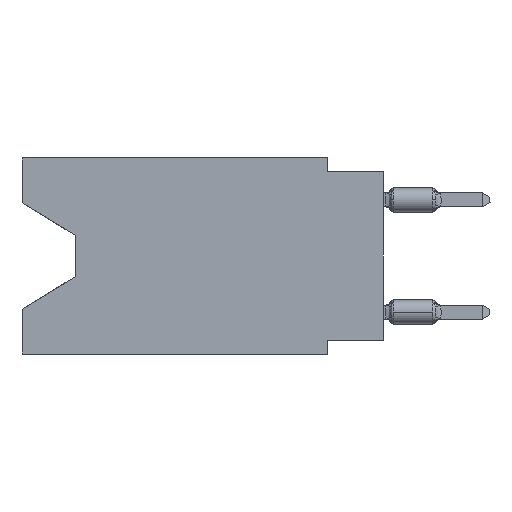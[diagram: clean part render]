
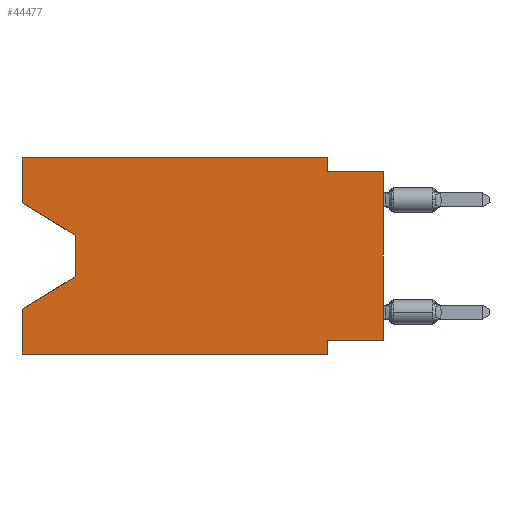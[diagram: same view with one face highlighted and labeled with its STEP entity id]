
A CAD part, left-side view. The second image highlights one B-rep face of the part: STEP entity #44477.
In plain terms, the highlighted planar face has unit normal (-1, 0, 0).
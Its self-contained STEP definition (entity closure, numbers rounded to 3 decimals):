
#53 = EDGE_CURVE ( 'NONE', #8936, #19838, #831, .T. ) ;
#192 = DIRECTION ( 'NONE',  ( 0., 0., 1. ) ) ;
#831 = LINE ( 'NONE', #1366, #6568 ) ;
#1353 = CARTESIAN_POINT ( 'NONE',  ( 0., 16.383, -2.038 ) ) ;
#1366 = CARTESIAN_POINT ( 'NONE',  ( 0., 16.383, -8.89 ) ) ;
#1413 = DIRECTION ( 'NONE',  ( 0., -1., 0. ) ) ;
#1794 = LINE ( 'NONE', #10398, #28857 ) ;
#2228 = VERTEX_POINT ( 'NONE', #4451 ) ;
#2782 = VERTEX_POINT ( 'NONE', #1353 ) ;
#2998 = DIRECTION ( 'NONE',  ( 0., 0., 1. ) ) ;
#3834 = FACE_OUTER_BOUND ( 'NONE', #28465, .T. ) ;
#4344 = VECTOR ( 'NONE', #18576, 1000. ) ;
#4451 = CARTESIAN_POINT ( 'NONE',  ( 0., 16.383, 0. ) ) ;
#4560 = LINE ( 'NONE', #53153, #26335 ) ;
#5319 = VECTOR ( 'NONE', #192, 1000. ) ;
#5365 = ORIENTED_EDGE ( 'NONE', *, *, #13552, .F. ) ;
#6349 = DIRECTION ( 'NONE',  ( 0., 0., -1. ) ) ;
#6568 = VECTOR ( 'NONE', #33372, 1000. ) ;
#6982 = VERTEX_POINT ( 'NONE', #52504 ) ;
#7954 = ORIENTED_EDGE ( 'NONE', *, *, #28000, .F. ) ;
#8135 = DIRECTION ( 'NONE',  ( 1., 0., 0. ) ) ;
#8501 = DIRECTION ( 'NONE',  ( 0., -1., 0. ) ) ;
#8926 = CARTESIAN_POINT ( 'NONE',  ( 0., 16.383, 0. ) ) ;
#8936 = VERTEX_POINT ( 'NONE', #34368 ) ;
#8953 = ORIENTED_EDGE ( 'NONE', *, *, #37714, .T. ) ;
#9332 = LINE ( 'NONE', #12830, #5319 ) ;
#10398 = CARTESIAN_POINT ( 'NONE',  ( 0., 2.54, -8.89 ) ) ;
#10589 = VECTOR ( 'NONE', #8501, 1000. ) ;
#11578 = CARTESIAN_POINT ( 'NONE',  ( 0., 13.97, -3.505 ) ) ;
#12590 = VERTEX_POINT ( 'NONE', #17169 ) ;
#12830 = CARTESIAN_POINT ( 'NONE',  ( 0., 16.383, 0. ) ) ;
#13552 = EDGE_CURVE ( 'NONE', #2782, #2228, #9332, .T. ) ;
#13594 = DIRECTION ( 'NONE',  ( 0., 0., -1. ) ) ;
#14296 = VERTEX_POINT ( 'NONE', #23752 ) ;
#14804 = ORIENTED_EDGE ( 'NONE', *, *, #40997, .F. ) ;
#15452 = ORIENTED_EDGE ( 'NONE', *, *, #26032, .T. ) ;
#15479 = CARTESIAN_POINT ( 'NONE',  ( 0., 13.97, -3.505 ) ) ;
#16416 = DIRECTION ( 'NONE',  ( 0., 0.855, -0.519 ) ) ;
#17169 = CARTESIAN_POINT ( 'NONE',  ( 0., 16.383, -6.852 ) ) ;
#17277 = PLANE ( 'NONE',  #29744 ) ;
#17378 = LINE ( 'NONE', #25703, #10589 ) ;
#17562 = LINE ( 'NONE', #26161, #45477 ) ;
#18576 = DIRECTION ( 'NONE',  ( 0., -0.855, -0.519 ) ) ;
#18681 = EDGE_CURVE ( 'NONE', #14296, #6982, #38583, .T. ) ;
#18889 = CARTESIAN_POINT ( 'NONE',  ( 0., 16.383, 0. ) ) ;
#19838 = VERTEX_POINT ( 'NONE', #30572 ) ;
#20214 = VERTEX_POINT ( 'NONE', #22178 ) ;
#20826 = EDGE_CURVE ( 'NONE', #35823, #30790, #28523, .T. ) ;
#21378 = ORIENTED_EDGE ( 'NONE', *, *, #30723, .F. ) ;
#22178 = CARTESIAN_POINT ( 'NONE',  ( 0., 0., -0.635 ) ) ;
#23124 = CARTESIAN_POINT ( 'NONE',  ( 0., 0., -8.255 ) ) ;
#23237 = ORIENTED_EDGE ( 'NONE', *, *, #18681, .F. ) ;
#23752 = CARTESIAN_POINT ( 'NONE',  ( 0., 2.54, 0. ) ) ;
#23971 = LINE ( 'NONE', #18889, #41963 ) ;
#25141 = EDGE_CURVE ( 'NONE', #2228, #14296, #17562, .T. ) ;
#25703 = CARTESIAN_POINT ( 'NONE',  ( 0., 0., -0.635 ) ) ;
#26032 = EDGE_CURVE ( 'NONE', #2782, #35823, #51874, .T. ) ;
#26161 = CARTESIAN_POINT ( 'NONE',  ( 0., 16.383, 0. ) ) ;
#26335 = VECTOR ( 'NONE', #16416, 1000. ) ;
#26837 = ORIENTED_EDGE ( 'NONE', *, *, #53, .T. ) ;
#26952 = VECTOR ( 'NONE', #41823, 1000. ) ;
#27309 = ORIENTED_EDGE ( 'NONE', *, *, #20826, .T. ) ;
#28000 = EDGE_CURVE ( 'NONE', #46604, #19838, #1794, .T. ) ;
#28158 = VECTOR ( 'NONE', #44898, 1000. ) ;
#28465 = EDGE_LOOP ( 'NONE', ( #15452, #27309, #51441, #14804, #26837, #7954, #21378, #8953, #45550, #23237, #42887, #5365 ) ) ;
#28523 = LINE ( 'NONE', #11578, #28158 ) ;
#28845 = DIRECTION ( 'NONE',  ( 0., 0., -1. ) ) ;
#28857 = VECTOR ( 'NONE', #6349, 1000. ) ;
#29477 = LINE ( 'NONE', #45852, #26952 ) ;
#29549 = VECTOR ( 'NONE', #34249, 1000. ) ;
#29744 = AXIS2_PLACEMENT_3D ( 'NONE', #8926, #8135, #28845 ) ;
#29955 = CARTESIAN_POINT ( 'NONE',  ( 0., 13.97, -5.385 ) ) ;
#30145 = EDGE_CURVE ( 'NONE', #6982, #20214, #17378, .T. ) ;
#30572 = CARTESIAN_POINT ( 'NONE',  ( 0., 2.54, -8.89 ) ) ;
#30664 = CARTESIAN_POINT ( 'NONE',  ( 0., 2.54, -8.255 ) ) ;
#30723 = EDGE_CURVE ( 'NONE', #31299, #46604, #42826, .T. ) ;
#30790 = VERTEX_POINT ( 'NONE', #29955 ) ;
#31299 = VERTEX_POINT ( 'NONE', #23124 ) ;
#33372 = DIRECTION ( 'NONE',  ( 0., -1., 0. ) ) ;
#34249 = DIRECTION ( 'NONE',  ( 0., 1., 0. ) ) ;
#34368 = CARTESIAN_POINT ( 'NONE',  ( 0., 16.383, -8.89 ) ) ;
#35615 = VECTOR ( 'NONE', #13594, 1000. ) ;
#35823 = VERTEX_POINT ( 'NONE', #15479 ) ;
#37714 = EDGE_CURVE ( 'NONE', #31299, #20214, #29477, .T. ) ;
#38583 = LINE ( 'NONE', #46906, #35615 ) ;
#38751 = CARTESIAN_POINT ( 'NONE',  ( 0., 16.383, -2.038 ) ) ;
#40997 = EDGE_CURVE ( 'NONE', #8936, #12590, #23971, .T. ) ;
#41823 = DIRECTION ( 'NONE',  ( 0., 0., 1. ) ) ;
#41963 = VECTOR ( 'NONE', #2998, 1000. ) ;
#42563 = CARTESIAN_POINT ( 'NONE',  ( 0., 0., -8.255 ) ) ;
#42826 = LINE ( 'NONE', #42563, #29549 ) ;
#42887 = ORIENTED_EDGE ( 'NONE', *, *, #25141, .F. ) ;
#44477 = ADVANCED_FACE ( 'NONE', ( #3834 ), #17277, .F. ) ;
#44774 = EDGE_CURVE ( 'NONE', #30790, #12590, #4560, .T. ) ;
#44898 = DIRECTION ( 'NONE',  ( 0., 0., -1. ) ) ;
#45477 = VECTOR ( 'NONE', #1413, 1000. ) ;
#45550 = ORIENTED_EDGE ( 'NONE', *, *, #30145, .F. ) ;
#45852 = CARTESIAN_POINT ( 'NONE',  ( 0., 0., 0. ) ) ;
#46604 = VERTEX_POINT ( 'NONE', #30664 ) ;
#46906 = CARTESIAN_POINT ( 'NONE',  ( 0., 2.54, 0. ) ) ;
#51441 = ORIENTED_EDGE ( 'NONE', *, *, #44774, .T. ) ;
#51874 = LINE ( 'NONE', #38751, #4344 ) ;
#52504 = CARTESIAN_POINT ( 'NONE',  ( 0., 2.54, -0.635 ) ) ;
#53153 = CARTESIAN_POINT ( 'NONE',  ( 0., 13.97, -5.385 ) ) ;
